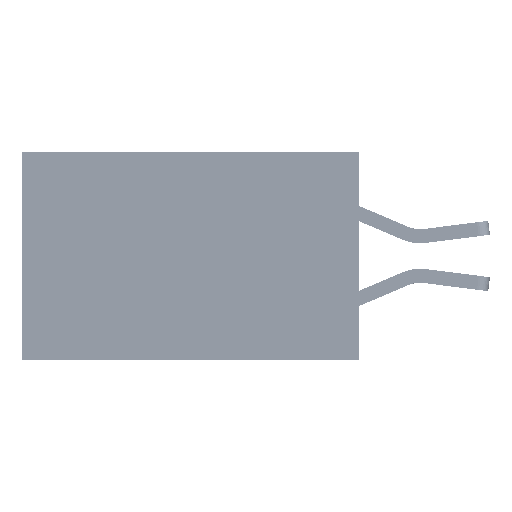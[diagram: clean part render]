
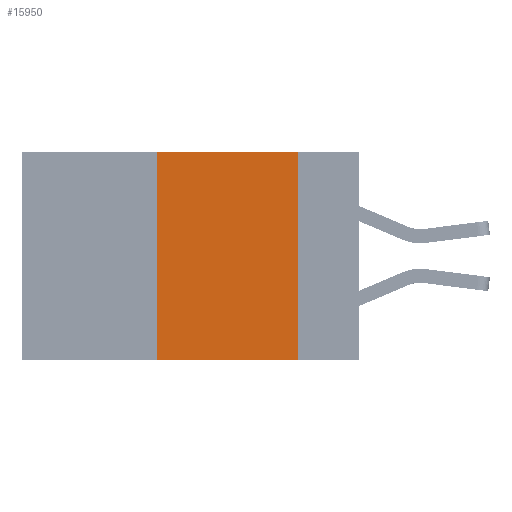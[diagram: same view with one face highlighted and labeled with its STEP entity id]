
A CAD part, left-side view. The second image highlights one B-rep face of the part: STEP entity #15950.
In plain terms, the highlighted planar face has unit normal (-1, 0, 0).
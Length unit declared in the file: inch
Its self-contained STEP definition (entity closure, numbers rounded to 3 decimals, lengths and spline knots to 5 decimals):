
#1727 = CARTESIAN_POINT ( 'NONE',  ( 0., 0.6, 0. ) ) ;
#1823 = PLANE ( 'NONE',  #6878 ) ;
#2735 = VERTEX_POINT ( 'NONE', #37083 ) ;
#4400 = CARTESIAN_POINT ( 'NONE',  ( 0., 0.6, -0.37 ) ) ;
#4700 = VERTEX_POINT ( 'NONE', #14774 ) ;
#6878 = AXIS2_PLACEMENT_3D ( 'NONE', #21676, #33466, #21943 ) ;
#7438 = EDGE_LOOP ( 'NONE', ( #8015, #22746, #23334, #15991 ) ) ;
#7947 = FACE_OUTER_BOUND ( 'NONE', #7438, .T. ) ;
#8015 = ORIENTED_EDGE ( 'NONE', *, *, #27073, .F. ) ;
#9435 = CARTESIAN_POINT ( 'NONE',  ( 0., 0.11, -0.37 ) ) ;
#9443 = VECTOR ( 'NONE', #29874, 39.37008 ) ;
#9997 = LINE ( 'NONE', #4400, #26631 ) ;
#10187 = DIRECTION ( 'NONE',  ( 0., -1., 0. ) ) ;
#14774 = CARTESIAN_POINT ( 'NONE',  ( 0., 0.36, -0.37 ) ) ;
#15576 = DIRECTION ( 'NONE',  ( 0., -1., 0. ) ) ;
#15950 = ADVANCED_FACE ( 'NONE', ( #7947 ), #1823, .F. ) ;
#15991 = ORIENTED_EDGE ( 'NONE', *, *, #33134, .T. ) ;
#17497 = LINE ( 'NONE', #1727, #35465 ) ;
#18112 = VECTOR ( 'NONE', #34025, 39.37008 ) ;
#18180 = CARTESIAN_POINT ( 'NONE',  ( 0., 0.11, 0. ) ) ;
#19639 = EDGE_CURVE ( 'NONE', #2735, #31923, #17497, .T. ) ;
#21676 = CARTESIAN_POINT ( 'NONE',  ( 0., 0.6, 0. ) ) ;
#21943 = DIRECTION ( 'NONE',  ( 0., 0., -1. ) ) ;
#22179 = LINE ( 'NONE', #33494, #18112 ) ;
#22746 = ORIENTED_EDGE ( 'NONE', *, *, #19639, .F. ) ;
#23334 = ORIENTED_EDGE ( 'NONE', *, *, #32746, .F. ) ;
#26416 = VERTEX_POINT ( 'NONE', #9435 ) ;
#26631 = VECTOR ( 'NONE', #10187, 39.37008 ) ;
#27073 = EDGE_CURVE ( 'NONE', #31923, #26416, #29685, .T. ) ;
#29685 = LINE ( 'NONE', #18180, #9443 ) ;
#29874 = DIRECTION ( 'NONE',  ( 0., 0., -1. ) ) ;
#31923 = VERTEX_POINT ( 'NONE', #33160 ) ;
#32746 = EDGE_CURVE ( 'NONE', #4700, #2735, #22179, .T. ) ;
#33134 = EDGE_CURVE ( 'NONE', #4700, #26416, #9997, .T. ) ;
#33160 = CARTESIAN_POINT ( 'NONE',  ( 0., 0.11, 0. ) ) ;
#33466 = DIRECTION ( 'NONE',  ( 1., 0., 0. ) ) ;
#33494 = CARTESIAN_POINT ( 'NONE',  ( 0., 0.36, 0. ) ) ;
#34025 = DIRECTION ( 'NONE',  ( 0., 0., 1. ) ) ;
#35465 = VECTOR ( 'NONE', #15576, 39.37008 ) ;
#37083 = CARTESIAN_POINT ( 'NONE',  ( 0., 0.36, 0. ) ) ;
